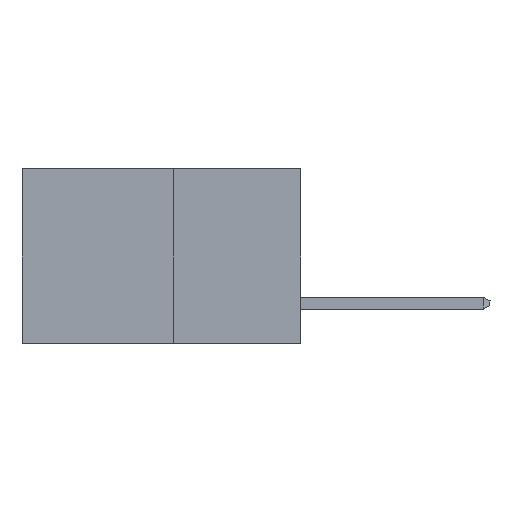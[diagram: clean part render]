
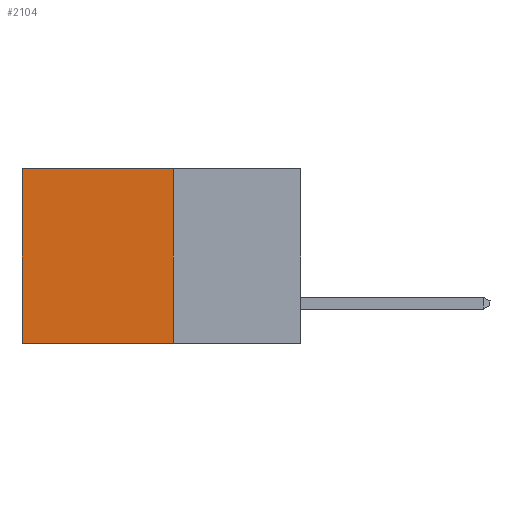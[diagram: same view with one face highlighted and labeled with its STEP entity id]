
A CAD part, left-side view. The second image highlights one B-rep face of the part: STEP entity #2104.
In plain terms, the highlighted planar face has unit normal (-1, 0, 0).
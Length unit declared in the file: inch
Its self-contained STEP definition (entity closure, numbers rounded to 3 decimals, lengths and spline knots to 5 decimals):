
#510 = CARTESIAN_POINT ( 'NONE',  ( 0.277, 0.59, -0.37 ) ) ;
#613 = VERTEX_POINT ( 'NONE', #5007 ) ;
#781 = DIRECTION ( 'NONE',  ( 0., 0., -1. ) ) ;
#1463 = EDGE_CURVE ( 'NONE', #613, #11668, #10055, .T. ) ;
#1820 = PLANE ( 'NONE',  #11570 ) ;
#2104 = ADVANCED_FACE ( 'NONE', ( #10673 ), #1820, .F. ) ;
#2646 = CARTESIAN_POINT ( 'NONE',  ( 0.277, 0.27, -0.37 ) ) ;
#4345 = LINE ( 'NONE', #4538, #15018 ) ;
#4538 = CARTESIAN_POINT ( 'NONE',  ( 0.277, 0.27, -0.37 ) ) ;
#4656 = CARTESIAN_POINT ( 'NONE',  ( 0.277, 0.27, 0. ) ) ;
#4929 = EDGE_LOOP ( 'NONE', ( #16125, #13124, #8527, #16341 ) ) ;
#5007 = CARTESIAN_POINT ( 'NONE',  ( 0.277, 0.27, 0. ) ) ;
#5182 = VECTOR ( 'NONE', #7814, 39.37008 ) ;
#5782 = CARTESIAN_POINT ( 'NONE',  ( 0.277, 0.59, -0.37 ) ) ;
#6508 = VECTOR ( 'NONE', #16014, 39.37008 ) ;
#7689 = CARTESIAN_POINT ( 'NONE',  ( 0.277, 0.27, -0.37 ) ) ;
#7814 = DIRECTION ( 'NONE',  ( 0., 1., 0. ) ) ;
#8023 = EDGE_CURVE ( 'NONE', #11668, #13006, #11241, .T. ) ;
#8300 = CARTESIAN_POINT ( 'NONE',  ( 0.277, 0.59, 0. ) ) ;
#8527 = ORIENTED_EDGE ( 'NONE', *, *, #11816, .F. ) ;
#10055 = LINE ( 'NONE', #4656, #6508 ) ;
#10255 = CARTESIAN_POINT ( 'NONE',  ( 0.277, 0.27, -0.37 ) ) ;
#10673 = FACE_OUTER_BOUND ( 'NONE', #4929, .T. ) ;
#11241 = LINE ( 'NONE', #5782, #14340 ) ;
#11570 = AXIS2_PLACEMENT_3D ( 'NONE', #2646, #16827, #781 ) ;
#11668 = VERTEX_POINT ( 'NONE', #8300 ) ;
#11816 = EDGE_CURVE ( 'NONE', #613, #17148, #4345, .T. ) ;
#12334 = LINE ( 'NONE', #7689, #5182 ) ;
#12648 = EDGE_CURVE ( 'NONE', #17148, #13006, #12334, .T. ) ;
#13006 = VERTEX_POINT ( 'NONE', #510 ) ;
#13124 = ORIENTED_EDGE ( 'NONE', *, *, #12648, .F. ) ;
#14340 = VECTOR ( 'NONE', #16377, 39.37008 ) ;
#15018 = VECTOR ( 'NONE', #15183, 39.37008 ) ;
#15183 = DIRECTION ( 'NONE',  ( 0., 0., -1. ) ) ;
#16014 = DIRECTION ( 'NONE',  ( 0., 1., 0. ) ) ;
#16125 = ORIENTED_EDGE ( 'NONE', *, *, #8023, .T. ) ;
#16341 = ORIENTED_EDGE ( 'NONE', *, *, #1463, .T. ) ;
#16377 = DIRECTION ( 'NONE',  ( 0., 0., -1. ) ) ;
#16827 = DIRECTION ( 'NONE',  ( 1., 0., 0. ) ) ;
#17148 = VERTEX_POINT ( 'NONE', #10255 ) ;
